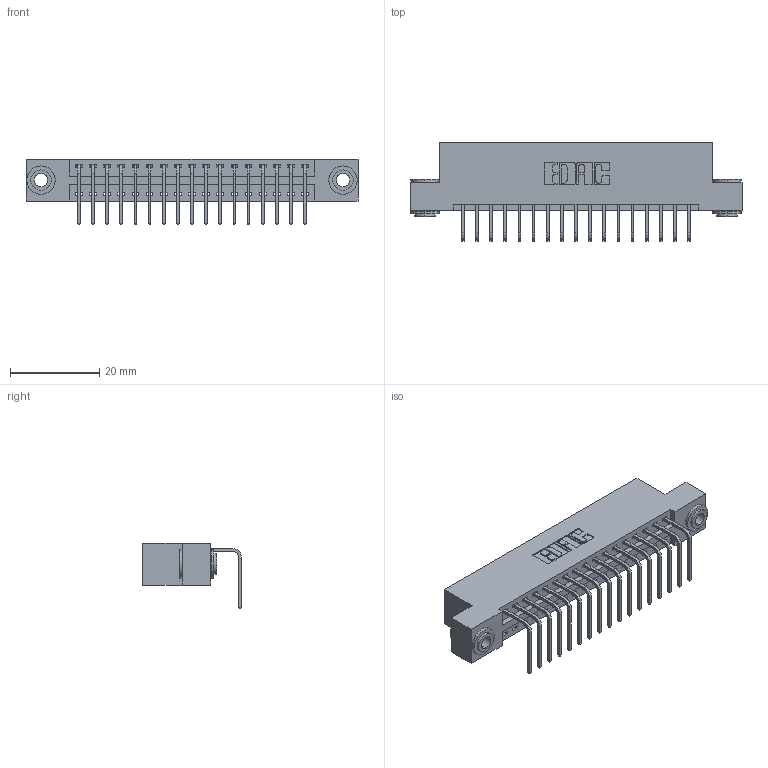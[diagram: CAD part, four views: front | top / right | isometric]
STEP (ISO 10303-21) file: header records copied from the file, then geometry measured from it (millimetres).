
FILE_DESCRIPTION (( 'STEP AP203' ), '1' );
FILE_NAME ('396-017-558-103.STEP', '2018-09-01T01:08:10', ( '' ), ( '' ), 'SwSTEP 2.0', 'SolidWorks 2016', '' );
FILE_SCHEMA (( 'CONFIG_CONTROL_DESIGN' ));
Length unit declared in the file: inch
Products named in the file (4): 346 Part_Flush Mounting Lugs - 0.156 Dia-TH; 345-292-001_558 Tail - 2; 345-250-002_345-250-002-102; 396-017-558-103
Assembly tree (20 placements, depth 2):
  396-017-558-103
    346 Part_Flush Mounting Lugs - 0.156 Dia-TH
    345-292-001_558 Tail - 2  x17
    345-250-002_345-250-002-102  x2
Bounding box: 74.55 x 22.16 x 14.73 mm (x, y, z)
Volume: 7039.8 mm3; surface area: 9086.1 mm2
Topology: 20 solids, 20 shells, 1180 faces, 3499 edges, 2306 vertices
Faces by surface type: plane 800, cylinder 372, cone 8
Entity records: 14650 total; most frequent: CARTESIAN_POINT 2498, ORIENTED_EDGE 2442, DIRECTION 2265, EDGE_CURVE 1221, LINE 997, VECTOR 997, VERTEX_POINT 810, AXIS2_PLACEMENT_3D 634
